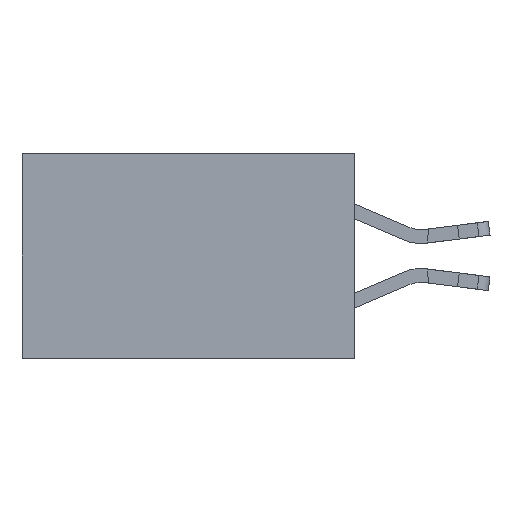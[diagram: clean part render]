
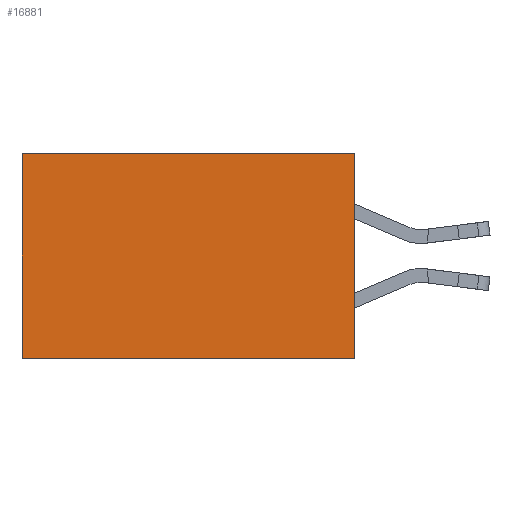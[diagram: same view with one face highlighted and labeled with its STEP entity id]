
A CAD part, left-side view. The second image highlights one B-rep face of the part: STEP entity #16881.
In plain terms, the highlighted planar face has unit normal (-1, 0, 0).
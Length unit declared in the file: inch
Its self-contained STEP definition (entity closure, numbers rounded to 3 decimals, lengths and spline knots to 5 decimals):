
#716 = CARTESIAN_POINT ( 'NONE',  ( 0.298, 0., 0. ) ) ;
#1056 = EDGE_LOOP ( 'NONE', ( #14432, #16131, #22179, #2901 ) ) ;
#1869 = CARTESIAN_POINT ( 'NONE',  ( 0.298, 0., -0.37 ) ) ;
#2824 = VERTEX_POINT ( 'NONE', #15320 ) ;
#2901 = ORIENTED_EDGE ( 'NONE', *, *, #22690, .T. ) ;
#2966 = DIRECTION ( 'NONE',  ( 0., 1., 0. ) ) ;
#4223 = EDGE_CURVE ( 'NONE', #12021, #8363, #6047, .T. ) ;
#4734 = PLANE ( 'NONE',  #11098 ) ;
#5897 = CARTESIAN_POINT ( 'NONE',  ( 0.298, 0.6, -0.37 ) ) ;
#6047 = LINE ( 'NONE', #9861, #11064 ) ;
#8363 = VERTEX_POINT ( 'NONE', #5897 ) ;
#8939 = VECTOR ( 'NONE', #16785, 39.37008 ) ;
#9026 = DIRECTION ( 'NONE',  ( 0., 0., -1. ) ) ;
#9518 = VECTOR ( 'NONE', #2966, 39.37008 ) ;
#9861 = CARTESIAN_POINT ( 'NONE',  ( 0.298, 0.6, 0. ) ) ;
#11064 = VECTOR ( 'NONE', #18974, 39.37008 ) ;
#11098 = AXIS2_PLACEMENT_3D ( 'NONE', #19613, #21726, #9026 ) ;
#12021 = VERTEX_POINT ( 'NONE', #26144 ) ;
#13816 = CARTESIAN_POINT ( 'NONE',  ( 0.298, 0., 0. ) ) ;
#14106 = CARTESIAN_POINT ( 'NONE',  ( 0.298, 0., 0. ) ) ;
#14432 = ORIENTED_EDGE ( 'NONE', *, *, #4223, .T. ) ;
#15189 = LINE ( 'NONE', #716, #9518 ) ;
#15320 = CARTESIAN_POINT ( 'NONE',  ( 0.298, 0., -0.37 ) ) ;
#15867 = DIRECTION ( 'NONE',  ( 0., 0., -1. ) ) ;
#15952 = EDGE_CURVE ( 'NONE', #2824, #8363, #20224, .T. ) ;
#16131 = ORIENTED_EDGE ( 'NONE', *, *, #15952, .F. ) ;
#16785 = DIRECTION ( 'NONE',  ( 0., 1., 0. ) ) ;
#16881 = ADVANCED_FACE ( 'NONE', ( #24450 ), #4734, .F. ) ;
#18443 = VERTEX_POINT ( 'NONE', #14106 ) ;
#18974 = DIRECTION ( 'NONE',  ( 0., 0., -1. ) ) ;
#19613 = CARTESIAN_POINT ( 'NONE',  ( 0.298, 0., 0. ) ) ;
#20224 = LINE ( 'NONE', #1869, #8939 ) ;
#21137 = LINE ( 'NONE', #13816, #26058 ) ;
#21726 = DIRECTION ( 'NONE',  ( 1., 0., 0. ) ) ;
#22179 = ORIENTED_EDGE ( 'NONE', *, *, #26332, .F. ) ;
#22690 = EDGE_CURVE ( 'NONE', #18443, #12021, #15189, .T. ) ;
#24450 = FACE_OUTER_BOUND ( 'NONE', #1056, .T. ) ;
#26058 = VECTOR ( 'NONE', #15867, 39.37008 ) ;
#26144 = CARTESIAN_POINT ( 'NONE',  ( 0.298, 0.6, 0. ) ) ;
#26332 = EDGE_CURVE ( 'NONE', #18443, #2824, #21137, .T. ) ;
